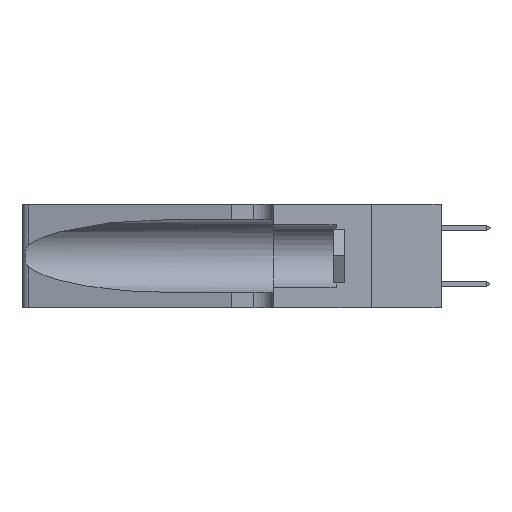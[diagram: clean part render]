
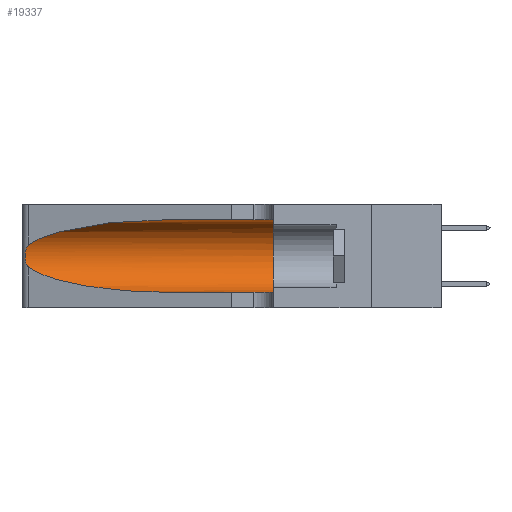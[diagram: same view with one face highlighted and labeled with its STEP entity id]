
A CAD part, left-side view. The second image highlights one B-rep face of the part: STEP entity #19337.
In plain terms, the highlighted cylindrical face has radius 3.308 mm (diameter 6.617 mm), a partial arc.
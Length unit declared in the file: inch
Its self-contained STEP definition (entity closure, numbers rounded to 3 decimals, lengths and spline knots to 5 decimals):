
#57 = CYLINDRICAL_SURFACE ( 'NONE', #8167, 0.13025 ) ;
#497 = ORIENTED_EDGE ( 'NONE', *, *, #14038, .T. ) ;
#584 = CARTESIAN_POINT ( 'NONE',  ( 0.25487, 1.22718, 0.22369 ) ) ;
#611 = CARTESIAN_POINT ( 'NONE',  ( 0.1305, 1.61858, 0.05475 ) ) ;
#713 = CARTESIAN_POINT ( 'NONE',  ( 0.25789, 1.23486, 0.15765 ) ) ;
#740 = LINE ( 'NONE', #611, #33947 ) ;
#918 = EDGE_CURVE ( 'NONE', #23567, #6194, #34273, .T. ) ;
#1188 =( BOUNDED_CURVE ( )  B_SPLINE_CURVE ( 3, ( #2158, #5305, #27164, #8466 ),
 .UNSPECIFIED., .F., .T. ) 
 B_SPLINE_CURVE_WITH_KNOTS ( ( 4, 4 ),
 ( 1.5708, 2.84003 ),
 .UNSPECIFIED. ) 
 CURVE ( )  GEOMETRIC_REPRESENTATION_ITEM ( )  RATIONAL_B_SPLINE_CURVE ( ( 1., 0.87, 0.87, 1. ) ) 
 REPRESENTATION_ITEM ( '' )  );
#1428 = CARTESIAN_POINT ( 'NONE',  ( 0.1305, 1.61858, 0.185 ) ) ;
#1703 = VERTEX_POINT ( 'NONE', #23289 ) ;
#2158 = CARTESIAN_POINT ( 'NONE',  ( 0.1305, 0.72297, 0.31525 ) ) ;
#2184 = VERTEX_POINT ( 'NONE', #28435 ) ;
#3857 = CARTESIAN_POINT ( 'NONE',  ( 0.25555, 1.22993, 0.14849 ) ) ;
#4618 = EDGE_CURVE ( 'NONE', #1703, #23567, #5254, .T. ) ;
#5254 = B_SPLINE_CURVE_WITH_KNOTS ( 'NONE', 3,
 ( #584, #16166, #28718, #10026, #31848, #13169, #35005, #16296, #38140, #19444, #713, #22580, #3857, #25733 ),
 .UNSPECIFIED., .F., .F.,
 ( 4, 2, 2, 2, 2, 2, 4 ),
 ( 0., 0.00027, 0.00053, 0.00107, 0.0016, 0.00187, 0.00214 ),
 .UNSPECIFIED. ) ;
#5305 = CARTESIAN_POINT ( 'NONE',  ( 0.18966, 0.96281, 0.31525 ) ) ;
#5551 = VERTEX_POINT ( 'NONE', #14318 ) ;
#6194 = VERTEX_POINT ( 'NONE', #17553 ) ;
#7157 = CARTESIAN_POINT ( 'NONE',  ( 0.25487, 1.22718, 0.14631 ) ) ;
#8167 = AXIS2_PLACEMENT_3D ( 'NONE', #1428, #30125, #11412 ) ;
#8466 = CARTESIAN_POINT ( 'NONE',  ( 0.25487, 1.22718, 0.22369 ) ) ;
#10026 = CARTESIAN_POINT ( 'NONE',  ( 0.25787, 1.23484, 0.2124 ) ) ;
#10201 = ORIENTED_EDGE ( 'NONE', *, *, #31938, .T. ) ;
#11023 = EDGE_CURVE ( 'NONE', #5551, #2184, #26489, .T. ) ;
#11412 = DIRECTION ( 'NONE',  ( 0., 0., -1. ) ) ;
#13169 = CARTESIAN_POINT ( 'NONE',  ( 0.26018, 1.23835, 0.19895 ) ) ;
#13523 = CARTESIAN_POINT ( 'NONE',  ( 0.18966, 0.96281, 0.05475 ) ) ;
#14038 = EDGE_CURVE ( 'NONE', #30088, #1703, #1188, .T. ) ;
#14318 = CARTESIAN_POINT ( 'NONE',  ( 0.1305, 0.35, 0.31525 ) ) ;
#15302 = VECTOR ( 'NONE', #22121, 39.37008 ) ;
#15653 = EDGE_CURVE ( 'NONE', #30088, #5551, #40237, .T. ) ;
#16166 = CARTESIAN_POINT ( 'NONE',  ( 0.25555, 1.22994, 0.2215 ) ) ;
#16296 = CARTESIAN_POINT ( 'NONE',  ( 0.26075, 1.23896, 0.178 ) ) ;
#16663 = CARTESIAN_POINT ( 'NONE',  ( 0.25487, 1.22718, 0.14631 ) ) ;
#16694 = FACE_OUTER_BOUND ( 'NONE', #20599, .T. ) ;
#17216 = DIRECTION ( 'NONE',  ( 0., 1., 0. ) ) ;
#17553 = CARTESIAN_POINT ( 'NONE',  ( 0.1305, 0.72297, 0.05475 ) ) ;
#19255 = ORIENTED_EDGE ( 'NONE', *, *, #15653, .F. ) ;
#19334 = ORIENTED_EDGE ( 'NONE', *, *, #11023, .F. ) ;
#19337 = ADVANCED_FACE ( 'NONE', ( #16694 ), #57, .F. ) ;
#19444 = CARTESIAN_POINT ( 'NONE',  ( 0.25856, 1.23593, 0.16098 ) ) ;
#20599 = EDGE_LOOP ( 'NONE', ( #497, #34223, #32344, #10201, #19334, #19255 ) ) ;
#22121 = DIRECTION ( 'NONE',  ( 0., -1., 0. ) ) ;
#22580 = CARTESIAN_POINT ( 'NONE',  ( 0.25639, 1.23186, 0.15144 ) ) ;
#23289 = CARTESIAN_POINT ( 'NONE',  ( 0.25487, 1.22718, 0.22369 ) ) ;
#23567 = VERTEX_POINT ( 'NONE', #7157 ) ;
#25733 = CARTESIAN_POINT ( 'NONE',  ( 0.25487, 1.22718, 0.14631 ) ) ;
#25948 = CARTESIAN_POINT ( 'NONE',  ( 0.2373, 1.15595, 0.08982 ) ) ;
#26489 = CIRCLE ( 'NONE', #37881, 0.13025 ) ;
#27164 = CARTESIAN_POINT ( 'NONE',  ( 0.2373, 1.15595, 0.28018 ) ) ;
#28435 = CARTESIAN_POINT ( 'NONE',  ( 0.1305, 0.35, 0.05475 ) ) ;
#28718 = CARTESIAN_POINT ( 'NONE',  ( 0.25639, 1.23184, 0.21858 ) ) ;
#28748 = DIRECTION ( 'NONE',  ( 0., -1., 0. ) ) ;
#30088 = VERTEX_POINT ( 'NONE', #31417 ) ;
#30125 = DIRECTION ( 'NONE',  ( 0., -1., 0. ) ) ;
#31417 = CARTESIAN_POINT ( 'NONE',  ( 0.1305, 0.72297, 0.31525 ) ) ;
#31534 = CARTESIAN_POINT ( 'NONE',  ( 0.1305, 1.61858, 0.31525 ) ) ;
#31848 = CARTESIAN_POINT ( 'NONE',  ( 0.25854, 1.2359, 0.20912 ) ) ;
#31938 = EDGE_CURVE ( 'NONE', #6194, #2184, #740, .T. ) ;
#32344 = ORIENTED_EDGE ( 'NONE', *, *, #918, .T. ) ;
#33947 = VECTOR ( 'NONE', #28748, 39.37008 ) ;
#34223 = ORIENTED_EDGE ( 'NONE', *, *, #4618, .T. ) ;
#34273 =( BOUNDED_CURVE ( )  B_SPLINE_CURVE ( 3, ( #16663, #25948, #13523, #38503 ),
 .UNSPECIFIED., .F., .T. ) 
 B_SPLINE_CURVE_WITH_KNOTS ( ( 4, 4 ),
 ( 3.44316, 4.71239 ),
 .UNSPECIFIED. ) 
 CURVE ( )  GEOMETRIC_REPRESENTATION_ITEM ( )  RATIONAL_B_SPLINE_CURVE ( ( 1., 0.87, 0.87, 1. ) ) 
 REPRESENTATION_ITEM ( '' )  );
#35005 = CARTESIAN_POINT ( 'NONE',  ( 0.26075, 1.23896, 0.19203 ) ) ;
#35917 = CARTESIAN_POINT ( 'NONE',  ( 0.1305, 0.35, 0.185 ) ) ;
#37881 = AXIS2_PLACEMENT_3D ( 'NONE', #35917, #17216, #39042 ) ;
#38140 = CARTESIAN_POINT ( 'NONE',  ( 0.26017, 1.23833, 0.17102 ) ) ;
#38503 = CARTESIAN_POINT ( 'NONE',  ( 0.1305, 0.72297, 0.05475 ) ) ;
#39042 = DIRECTION ( 'NONE',  ( 0., 0., 1. ) ) ;
#40237 = LINE ( 'NONE', #31534, #15302 ) ;
